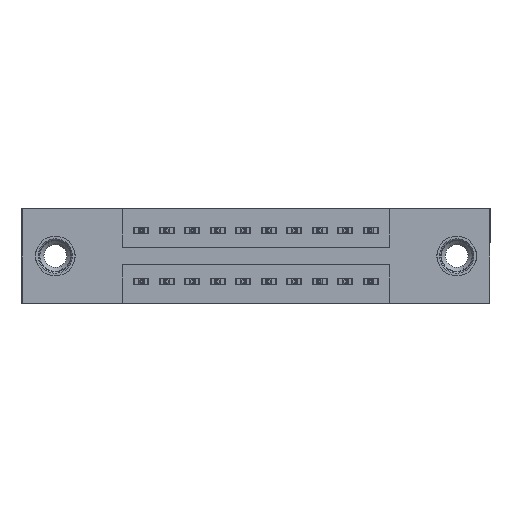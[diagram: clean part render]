
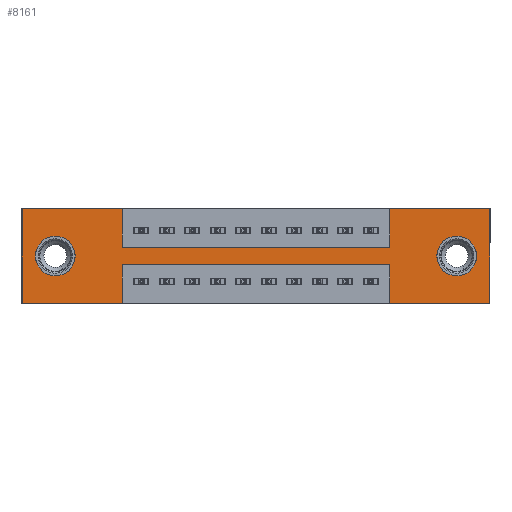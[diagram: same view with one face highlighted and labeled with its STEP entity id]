
A CAD part, front view. The second image highlights one B-rep face of the part: STEP entity #8161.
In plain terms, the highlighted planar face has unit normal (0, -1, 0).
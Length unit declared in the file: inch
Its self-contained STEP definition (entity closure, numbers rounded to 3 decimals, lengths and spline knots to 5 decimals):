
#92 = DIRECTION ( 'NONE',  ( -1., 0., 0. ) ) ;
#255 = AXIS2_PLACEMENT_3D ( 'NONE', #5331, #14402, #6648 ) ;
#308 = AXIS2_PLACEMENT_3D ( 'NONE', #14834, #9307, #1353 ) ;
#475 = EDGE_CURVE ( 'NONE', #2217, #12469, #12120, .T. ) ;
#560 = DIRECTION ( 'NONE',  ( 1., 0., 0. ) ) ;
#601 = CARTESIAN_POINT ( 'NONE',  ( 1.4425, 0., -0.22 ) ) ;
#966 = CARTESIAN_POINT ( 'NONE',  ( 0., 0., -0.37 ) ) ;
#1040 = CARTESIAN_POINT ( 'NONE',  ( 1.705, 0., -0.185 ) ) ;
#1151 = CARTESIAN_POINT ( 'NONE',  ( 1.4425, 0., 0. ) ) ;
#1353 = DIRECTION ( 'NONE',  ( 0., 0., 1. ) ) ;
#1388 = ORIENTED_EDGE ( 'NONE', *, *, #475, .F. ) ;
#1609 = VECTOR ( 'NONE', #13990, 39.37008 ) ;
#1830 = LINE ( 'NONE', #4798, #4561 ) ;
#2025 = ORIENTED_EDGE ( 'NONE', *, *, #9131, .F. ) ;
#2069 = EDGE_CURVE ( 'NONE', #14693, #2907, #1830, .T. ) ;
#2217 = VERTEX_POINT ( 'NONE', #6030 ) ;
#2309 = EDGE_CURVE ( 'NONE', #12469, #14693, #5192, .T. ) ;
#2326 = LINE ( 'NONE', #13244, #15809 ) ;
#2348 = DIRECTION ( 'NONE',  ( 0., -1., 0. ) ) ;
#2356 = VERTEX_POINT ( 'NONE', #601 ) ;
#2407 = DIRECTION ( 'NONE',  ( 0., 0., -1. ) ) ;
#2602 = CIRCLE ( 'NONE', #255, 0.078 ) ;
#2650 = CIRCLE ( 'NONE', #10692, 0.078 ) ;
#2895 = VECTOR ( 'NONE', #15221, 39.37008 ) ;
#2907 = VERTEX_POINT ( 'NONE', #4991 ) ;
#2916 = VECTOR ( 'NONE', #3672, 39.37008 ) ;
#2959 = EDGE_CURVE ( 'NONE', #13337, #3059, #13497, .T. ) ;
#3009 = EDGE_CURVE ( 'NONE', #3059, #13337, #2650, .T. ) ;
#3020 = LINE ( 'NONE', #5924, #8813 ) ;
#3031 = CARTESIAN_POINT ( 'NONE',  ( 1.705, 0., -0.107 ) ) ;
#3040 = VERTEX_POINT ( 'NONE', #1151 ) ;
#3059 = VERTEX_POINT ( 'NONE', #10466 ) ;
#3132 = VECTOR ( 'NONE', #92, 39.37008 ) ;
#3435 = VECTOR ( 'NONE', #7135, 39.37008 ) ;
#3437 = VERTEX_POINT ( 'NONE', #16354 ) ;
#3672 = DIRECTION ( 'NONE',  ( 0., 0., 1. ) ) ;
#3878 = CARTESIAN_POINT ( 'NONE',  ( 0.3925, 0., 0. ) ) ;
#3994 = EDGE_LOOP ( 'NONE', ( #13690, #14499, #8257, #2025, #5998, #12897, #13705, #4549, #8061, #1388, #15329, #5805 ) ) ;
#4085 = CARTESIAN_POINT ( 'NONE',  ( 0.13, 0., -0.107 ) ) ;
#4473 = EDGE_CURVE ( 'NONE', #6767, #9707, #6148, .T. ) ;
#4522 = EDGE_CURVE ( 'NONE', #3437, #5615, #3020, .T. ) ;
#4530 = CARTESIAN_POINT ( 'NONE',  ( 1.835, 0., 0. ) ) ;
#4549 = ORIENTED_EDGE ( 'NONE', *, *, #2069, .F. ) ;
#4561 = VECTOR ( 'NONE', #6339, 39.37008 ) ;
#4798 = CARTESIAN_POINT ( 'NONE',  ( 0.3925, 0., -0.15 ) ) ;
#4933 = VERTEX_POINT ( 'NONE', #9286 ) ;
#4991 = CARTESIAN_POINT ( 'NONE',  ( 1.4425, 0., -0.15 ) ) ;
#5068 = DIRECTION ( 'NONE',  ( 0., 0., 1. ) ) ;
#5192 = LINE ( 'NONE', #14028, #1609 ) ;
#5219 = VECTOR ( 'NONE', #11956, 39.37008 ) ;
#5331 = CARTESIAN_POINT ( 'NONE',  ( 0.13, 0., -0.185 ) ) ;
#5340 = CARTESIAN_POINT ( 'NONE',  ( 1.835, 0., -0.37 ) ) ;
#5460 = VERTEX_POINT ( 'NONE', #4085 ) ;
#5615 = VERTEX_POINT ( 'NONE', #8794 ) ;
#5704 = CARTESIAN_POINT ( 'NONE',  ( 1.4425, 0., -0.37 ) ) ;
#5805 = ORIENTED_EDGE ( 'NONE', *, *, #4522, .F. ) ;
#5924 = CARTESIAN_POINT ( 'NONE',  ( 0., 0., -0.37 ) ) ;
#5998 = ORIENTED_EDGE ( 'NONE', *, *, #4473, .F. ) ;
#6030 = CARTESIAN_POINT ( 'NONE',  ( 0., 0., 0. ) ) ;
#6148 = LINE ( 'NONE', #4530, #3435 ) ;
#6267 = CIRCLE ( 'NONE', #308, 0.078 ) ;
#6339 = DIRECTION ( 'NONE',  ( 1., 0., 0. ) ) ;
#6438 = LINE ( 'NONE', #12607, #2895 ) ;
#6460 = LINE ( 'NONE', #16638, #2916 ) ;
#6491 = DIRECTION ( 'NONE',  ( 0., 1., 0. ) ) ;
#6505 = AXIS2_PLACEMENT_3D ( 'NONE', #966, #2348, #11519 ) ;
#6575 = LINE ( 'NONE', #9572, #13063 ) ;
#6648 = DIRECTION ( 'NONE',  ( 0., 0., 1. ) ) ;
#6767 = VERTEX_POINT ( 'NONE', #8524 ) ;
#6793 = CARTESIAN_POINT ( 'NONE',  ( 0., 0., -0.37 ) ) ;
#6815 = ORIENTED_EDGE ( 'NONE', *, *, #13202, .T. ) ;
#7078 = EDGE_CURVE ( 'NONE', #5460, #14808, #6267, .T. ) ;
#7135 = DIRECTION ( 'NONE',  ( 0., 0., -1. ) ) ;
#7247 = DIRECTION ( 'NONE',  ( -1., 0., 0. ) ) ;
#8011 = LINE ( 'NONE', #8547, #15276 ) ;
#8061 = ORIENTED_EDGE ( 'NONE', *, *, #2309, .F. ) ;
#8161 = ADVANCED_FACE ( 'NONE', ( #10575, #13187, #10169 ), #8950, .T. ) ;
#8257 = ORIENTED_EDGE ( 'NONE', *, *, #14988, .F. ) ;
#8267 = DIRECTION ( 'NONE',  ( -1., 0., 0. ) ) ;
#8524 = CARTESIAN_POINT ( 'NONE',  ( 1.835, 0., 0. ) ) ;
#8547 = CARTESIAN_POINT ( 'NONE',  ( 0., 0., 0. ) ) ;
#8794 = CARTESIAN_POINT ( 'NONE',  ( 0., 0., -0.37 ) ) ;
#8813 = VECTOR ( 'NONE', #7247, 39.37008 ) ;
#8860 = CARTESIAN_POINT ( 'NONE',  ( 0.13, 0., -0.263 ) ) ;
#8950 = PLANE ( 'NONE',  #6505 ) ;
#8976 = AXIS2_PLACEMENT_3D ( 'NONE', #1040, #10297, #2407 ) ;
#9131 = EDGE_CURVE ( 'NONE', #9707, #10739, #10132, .T. ) ;
#9286 = CARTESIAN_POINT ( 'NONE',  ( 0.3925, 0., -0.22 ) ) ;
#9307 = DIRECTION ( 'NONE',  ( 0., 1., 0. ) ) ;
#9572 = CARTESIAN_POINT ( 'NONE',  ( 0.3925, 0., -0.22 ) ) ;
#9707 = VERTEX_POINT ( 'NONE', #5340 ) ;
#10069 = EDGE_CURVE ( 'NONE', #5615, #2217, #6460, .T. ) ;
#10132 = LINE ( 'NONE', #6793, #3132 ) ;
#10169 = FACE_OUTER_BOUND ( 'NONE', #3994, .T. ) ;
#10297 = DIRECTION ( 'NONE',  ( 0., 1., 0. ) ) ;
#10466 = CARTESIAN_POINT ( 'NONE',  ( 1.705, 0., -0.263 ) ) ;
#10575 = FACE_BOUND ( 'NONE', #14678, .T. ) ;
#10692 = AXIS2_PLACEMENT_3D ( 'NONE', #14247, #6491, #15539 ) ;
#10739 = VERTEX_POINT ( 'NONE', #5704 ) ;
#10922 = CARTESIAN_POINT ( 'NONE',  ( 0., 0., 0. ) ) ;
#11519 = DIRECTION ( 'NONE',  ( 0., 0., -1. ) ) ;
#11695 = LINE ( 'NONE', #14146, #14737 ) ;
#11956 = DIRECTION ( 'NONE',  ( 1., 0., 0. ) ) ;
#12065 = ORIENTED_EDGE ( 'NONE', *, *, #7078, .T. ) ;
#12120 = LINE ( 'NONE', #10922, #5219 ) ;
#12261 = ORIENTED_EDGE ( 'NONE', *, *, #3009, .T. ) ;
#12469 = VERTEX_POINT ( 'NONE', #3878 ) ;
#12607 = CARTESIAN_POINT ( 'NONE',  ( 0.3925, 0., -0.37 ) ) ;
#12617 = EDGE_LOOP ( 'NONE', ( #12065, #6815 ) ) ;
#12640 = ORIENTED_EDGE ( 'NONE', *, *, #2959, .T. ) ;
#12706 = EDGE_CURVE ( 'NONE', #2356, #4933, #6575, .T. ) ;
#12839 = EDGE_CURVE ( 'NONE', #3040, #6767, #8011, .T. ) ;
#12897 = ORIENTED_EDGE ( 'NONE', *, *, #12839, .F. ) ;
#13063 = VECTOR ( 'NONE', #8267, 39.37008 ) ;
#13187 = FACE_BOUND ( 'NONE', #12617, .T. ) ;
#13202 = EDGE_CURVE ( 'NONE', #14808, #5460, #2602, .T. ) ;
#13244 = CARTESIAN_POINT ( 'NONE',  ( 1.4425, 0., -0.37 ) ) ;
#13337 = VERTEX_POINT ( 'NONE', #3031 ) ;
#13497 = CIRCLE ( 'NONE', #8976, 0.078 ) ;
#13690 = ORIENTED_EDGE ( 'NONE', *, *, #16594, .F. ) ;
#13705 = ORIENTED_EDGE ( 'NONE', *, *, #16704, .F. ) ;
#13874 = CARTESIAN_POINT ( 'NONE',  ( 0.3925, 0., -0.15 ) ) ;
#13990 = DIRECTION ( 'NONE',  ( 0., 0., -1. ) ) ;
#14028 = CARTESIAN_POINT ( 'NONE',  ( 0.3925, 0., 0. ) ) ;
#14146 = CARTESIAN_POINT ( 'NONE',  ( 1.4425, 0., 0. ) ) ;
#14247 = CARTESIAN_POINT ( 'NONE',  ( 1.705, 0., -0.185 ) ) ;
#14402 = DIRECTION ( 'NONE',  ( 0., 1., 0. ) ) ;
#14499 = ORIENTED_EDGE ( 'NONE', *, *, #12706, .F. ) ;
#14542 = DIRECTION ( 'NONE',  ( 0., 0., 1. ) ) ;
#14678 = EDGE_LOOP ( 'NONE', ( #12640, #12261 ) ) ;
#14693 = VERTEX_POINT ( 'NONE', #13874 ) ;
#14737 = VECTOR ( 'NONE', #5068, 39.37008 ) ;
#14808 = VERTEX_POINT ( 'NONE', #8860 ) ;
#14834 = CARTESIAN_POINT ( 'NONE',  ( 0.13, 0., -0.185 ) ) ;
#14988 = EDGE_CURVE ( 'NONE', #10739, #2356, #2326, .T. ) ;
#15221 = DIRECTION ( 'NONE',  ( 0., 0., -1. ) ) ;
#15276 = VECTOR ( 'NONE', #560, 39.37008 ) ;
#15329 = ORIENTED_EDGE ( 'NONE', *, *, #10069, .F. ) ;
#15539 = DIRECTION ( 'NONE',  ( 0., 0., -1. ) ) ;
#15809 = VECTOR ( 'NONE', #14542, 39.37008 ) ;
#16354 = CARTESIAN_POINT ( 'NONE',  ( 0.3925, 0., -0.37 ) ) ;
#16594 = EDGE_CURVE ( 'NONE', #4933, #3437, #6438, .T. ) ;
#16638 = CARTESIAN_POINT ( 'NONE',  ( 0., 0., 0. ) ) ;
#16704 = EDGE_CURVE ( 'NONE', #2907, #3040, #11695, .T. ) ;
